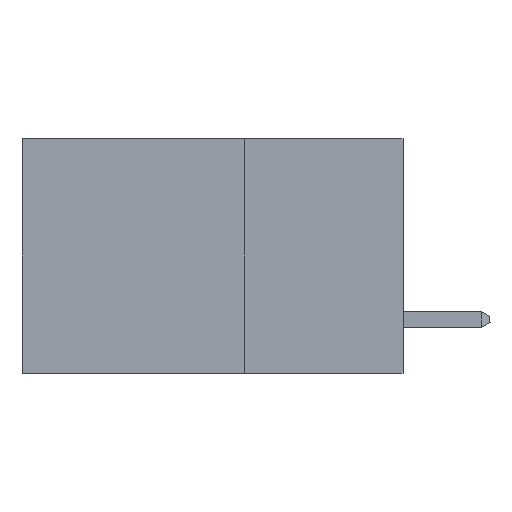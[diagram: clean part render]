
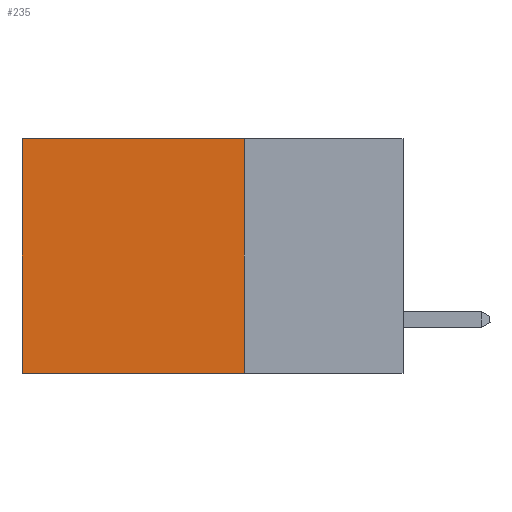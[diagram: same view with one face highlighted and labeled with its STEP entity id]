
A CAD part, left-side view. The second image highlights one B-rep face of the part: STEP entity #235.
In plain terms, the highlighted planar face has unit normal (-1, 0, 0).
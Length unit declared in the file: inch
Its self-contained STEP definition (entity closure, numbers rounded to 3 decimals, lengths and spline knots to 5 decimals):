
#116 = VERTEX_POINT ( 'NONE', #4896 ) ;
#191 = VECTOR ( 'NONE', #5249, 39.37008 ) ;
#235 = ADVANCED_FACE ( 'NONE', ( #7213 ), #10575, .F. ) ;
#809 = CARTESIAN_POINT ( 'NONE',  ( 0.2875, 0.6, -0.37 ) ) ;
#1127 = CARTESIAN_POINT ( 'NONE',  ( 0.2875, 0.6, 0. ) ) ;
#1341 = EDGE_CURVE ( 'NONE', #116, #10838, #2208, .T. ) ;
#1930 = EDGE_CURVE ( 'NONE', #4404, #116, #5991, .T. ) ;
#2208 = LINE ( 'NONE', #4264, #4314 ) ;
#2299 = CARTESIAN_POINT ( 'NONE',  ( 0.2875, 0.25, 0. ) ) ;
#2816 = CARTESIAN_POINT ( 'NONE',  ( 0.2875, 0.25, 0. ) ) ;
#2862 = VERTEX_POINT ( 'NONE', #5293 ) ;
#3454 = EDGE_LOOP ( 'NONE', ( #7458, #7926, #7790, #9875 ) ) ;
#3575 = VECTOR ( 'NONE', #6624, 39.37008 ) ;
#4264 = CARTESIAN_POINT ( 'NONE',  ( 0.2875, 0.25, -0.37 ) ) ;
#4314 = VECTOR ( 'NONE', #11998, 39.37008 ) ;
#4404 = VERTEX_POINT ( 'NONE', #2299 ) ;
#4834 = EDGE_CURVE ( 'NONE', #2862, #10838, #12236, .T. ) ;
#4896 = CARTESIAN_POINT ( 'NONE',  ( 0.2875, 0.25, -0.37 ) ) ;
#5017 = DIRECTION ( 'NONE',  ( 0., 1., 0. ) ) ;
#5249 = DIRECTION ( 'NONE',  ( 0., 0., -1. ) ) ;
#5293 = CARTESIAN_POINT ( 'NONE',  ( 0.2875, 0.6, 0. ) ) ;
#5765 = DIRECTION ( 'NONE',  ( 0., 0., -1. ) ) ;
#5804 = DIRECTION ( 'NONE',  ( 1., 0., 0. ) ) ;
#5902 = CARTESIAN_POINT ( 'NONE',  ( 0.2875, 0.25, 0. ) ) ;
#5991 = LINE ( 'NONE', #10248, #3575 ) ;
#6184 = LINE ( 'NONE', #5902, #7380 ) ;
#6624 = DIRECTION ( 'NONE',  ( 0., 0., -1. ) ) ;
#7213 = FACE_OUTER_BOUND ( 'NONE', #3454, .T. ) ;
#7380 = VECTOR ( 'NONE', #5017, 39.37008 ) ;
#7458 = ORIENTED_EDGE ( 'NONE', *, *, #4834, .T. ) ;
#7790 = ORIENTED_EDGE ( 'NONE', *, *, #1930, .F. ) ;
#7926 = ORIENTED_EDGE ( 'NONE', *, *, #1341, .F. ) ;
#9875 = ORIENTED_EDGE ( 'NONE', *, *, #11671, .T. ) ;
#10248 = CARTESIAN_POINT ( 'NONE',  ( 0.2875, 0.25, 0. ) ) ;
#10575 = PLANE ( 'NONE',  #12010 ) ;
#10838 = VERTEX_POINT ( 'NONE', #809 ) ;
#11671 = EDGE_CURVE ( 'NONE', #4404, #2862, #6184, .T. ) ;
#11998 = DIRECTION ( 'NONE',  ( 0., 1., 0. ) ) ;
#12010 = AXIS2_PLACEMENT_3D ( 'NONE', #2816, #5804, #5765 ) ;
#12236 = LINE ( 'NONE', #1127, #191 ) ;
